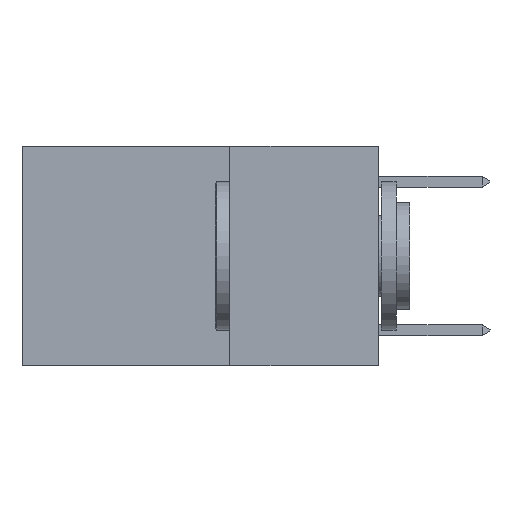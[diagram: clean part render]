
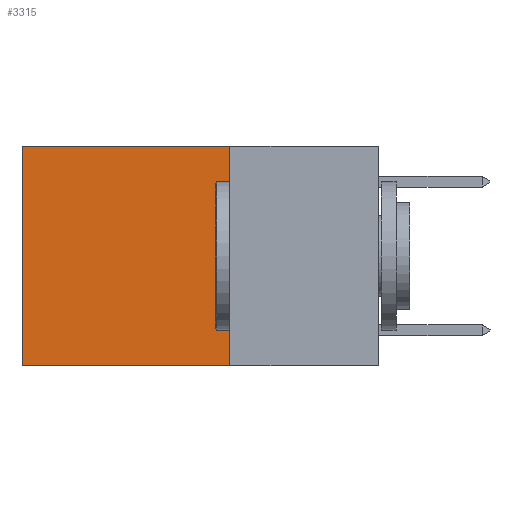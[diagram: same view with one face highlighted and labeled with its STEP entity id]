
A CAD part, left-side view. The second image highlights one B-rep face of the part: STEP entity #3315.
In plain terms, the highlighted planar face has unit normal (-1, 0, 0).
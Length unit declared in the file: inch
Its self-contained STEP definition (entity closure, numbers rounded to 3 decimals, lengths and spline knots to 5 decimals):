
#80 = VERTEX_POINT ( 'NONE', #13782 ) ;
#594 = CARTESIAN_POINT ( 'NONE',  ( 0.2625, 0.6, 0. ) ) ;
#632 = DIRECTION ( 'NONE',  ( 0., 0., -1. ) ) ;
#675 = ORIENTED_EDGE ( 'NONE', *, *, #16648, .F. ) ;
#1464 = CARTESIAN_POINT ( 'NONE',  ( 0.2625, 0.25, 0. ) ) ;
#3203 = LINE ( 'NONE', #1464, #3423 ) ;
#3315 = ADVANCED_FACE ( 'NONE', ( #8447 ), #7431, .F. ) ;
#3423 = VECTOR ( 'NONE', #4487, 39.37008 ) ;
#3438 = EDGE_CURVE ( 'NONE', #6169, #13949, #3203, .T. ) ;
#4160 = CARTESIAN_POINT ( 'NONE',  ( 0.2625, 0.25, 0. ) ) ;
#4360 = DIRECTION ( 'NONE',  ( 0., 0., -1. ) ) ;
#4487 = DIRECTION ( 'NONE',  ( 0., 1., 0. ) ) ;
#4561 = CARTESIAN_POINT ( 'NONE',  ( 0.2625, 0.25, 0. ) ) ;
#4775 = AXIS2_PLACEMENT_3D ( 'NONE', #4561, #8047, #632 ) ;
#5388 = VECTOR ( 'NONE', #4360, 39.37008 ) ;
#5966 = EDGE_LOOP ( 'NONE', ( #7899, #675, #13550, #6097 ) ) ;
#6069 = VECTOR ( 'NONE', #16225, 39.37008 ) ;
#6097 = ORIENTED_EDGE ( 'NONE', *, *, #3438, .T. ) ;
#6169 = VERTEX_POINT ( 'NONE', #4160 ) ;
#7431 = PLANE ( 'NONE',  #4775 ) ;
#7899 = ORIENTED_EDGE ( 'NONE', *, *, #11892, .T. ) ;
#8047 = DIRECTION ( 'NONE',  ( 1., 0., 0. ) ) ;
#8273 = DIRECTION ( 'NONE',  ( 0., 1., 0. ) ) ;
#8447 = FACE_OUTER_BOUND ( 'NONE', #5966, .T. ) ;
#8737 = VECTOR ( 'NONE', #8273, 39.37008 ) ;
#9148 = CARTESIAN_POINT ( 'NONE',  ( 0.2625, 0.6, 0. ) ) ;
#10414 = VERTEX_POINT ( 'NONE', #18700 ) ;
#10589 = LINE ( 'NONE', #9148, #6069 ) ;
#11214 = LINE ( 'NONE', #14181, #8737 ) ;
#11359 = EDGE_CURVE ( 'NONE', #6169, #80, #14937, .T. ) ;
#11892 = EDGE_CURVE ( 'NONE', #13949, #10414, #10589, .T. ) ;
#12528 = CARTESIAN_POINT ( 'NONE',  ( 0.2625, 0.25, 0. ) ) ;
#13550 = ORIENTED_EDGE ( 'NONE', *, *, #11359, .F. ) ;
#13782 = CARTESIAN_POINT ( 'NONE',  ( 0.2625, 0.25, -0.37 ) ) ;
#13949 = VERTEX_POINT ( 'NONE', #594 ) ;
#14181 = CARTESIAN_POINT ( 'NONE',  ( 0.2625, 0.25, -0.37 ) ) ;
#14937 = LINE ( 'NONE', #12528, #5388 ) ;
#16225 = DIRECTION ( 'NONE',  ( 0., 0., -1. ) ) ;
#16648 = EDGE_CURVE ( 'NONE', #80, #10414, #11214, .T. ) ;
#18700 = CARTESIAN_POINT ( 'NONE',  ( 0.2625, 0.6, -0.37 ) ) ;
